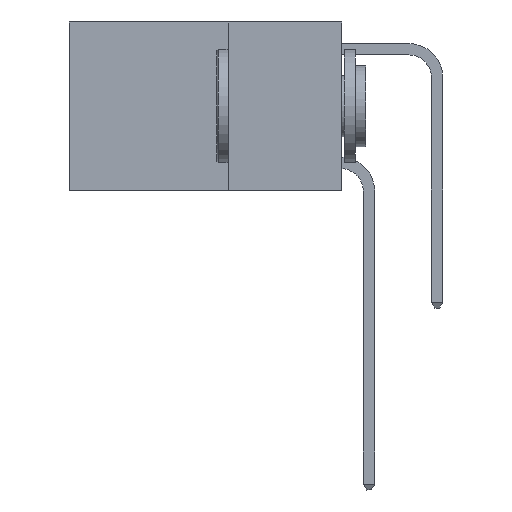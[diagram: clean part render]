
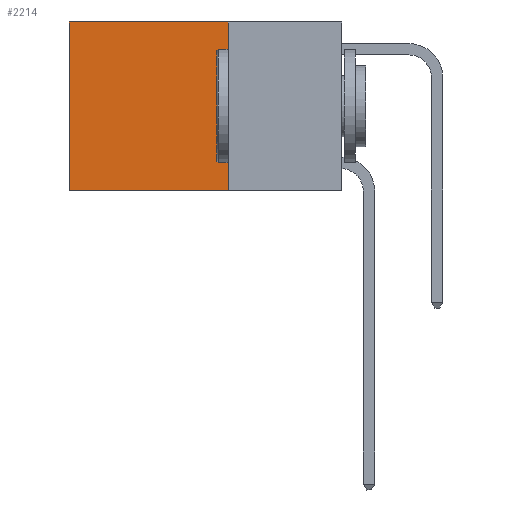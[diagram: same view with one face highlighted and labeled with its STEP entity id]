
A CAD part, left-side view. The second image highlights one B-rep face of the part: STEP entity #2214.
In plain terms, the highlighted planar face has unit normal (-1, 0, 0).
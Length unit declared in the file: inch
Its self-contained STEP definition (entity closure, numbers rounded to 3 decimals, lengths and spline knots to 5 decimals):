
#125 = CARTESIAN_POINT ( 'NONE',  ( 0.2625, 0.25, -0.37 ) ) ;
#917 = CARTESIAN_POINT ( 'NONE',  ( 0.2625, 0.25, 0. ) ) ;
#1165 = LINE ( 'NONE', #2291, #1263 ) ;
#1263 = VECTOR ( 'NONE', #8881, 39.37008 ) ;
#1786 = ORIENTED_EDGE ( 'NONE', *, *, #6537, .F. ) ;
#1971 = LINE ( 'NONE', #917, #6489 ) ;
#2214 = ADVANCED_FACE ( 'NONE', ( #12049 ), #8789, .F. ) ;
#2291 = CARTESIAN_POINT ( 'NONE',  ( 0.2625, 0.25, 0. ) ) ;
#2341 = ORIENTED_EDGE ( 'NONE', *, *, #13356, .T. ) ;
#2422 = CARTESIAN_POINT ( 'NONE',  ( 0.2625, 0.6, 0. ) ) ;
#2552 = VERTEX_POINT ( 'NONE', #7772 ) ;
#3150 = DIRECTION ( 'NONE',  ( 0., 0., -1. ) ) ;
#3165 = AXIS2_PLACEMENT_3D ( 'NONE', #13238, #5432, #12272 ) ;
#4122 = EDGE_CURVE ( 'NONE', #11083, #5513, #1971, .T. ) ;
#4127 = VECTOR ( 'NONE', #8019, 39.37008 ) ;
#4864 = CARTESIAN_POINT ( 'NONE',  ( 0.2625, 0.25, -0.37 ) ) ;
#4879 = LINE ( 'NONE', #2422, #11373 ) ;
#5432 = DIRECTION ( 'NONE',  ( 1., 0., 0. ) ) ;
#5513 = VERTEX_POINT ( 'NONE', #125 ) ;
#6039 = CARTESIAN_POINT ( 'NONE',  ( 0.2625, 0.25, 0. ) ) ;
#6049 = ORIENTED_EDGE ( 'NONE', *, *, #4122, .F. ) ;
#6489 = VECTOR ( 'NONE', #3150, 39.37008 ) ;
#6537 = EDGE_CURVE ( 'NONE', #5513, #2552, #9519, .T. ) ;
#7772 = CARTESIAN_POINT ( 'NONE',  ( 0.2625, 0.6, -0.37 ) ) ;
#7833 = CARTESIAN_POINT ( 'NONE',  ( 0.2625, 0.6, 0. ) ) ;
#8019 = DIRECTION ( 'NONE',  ( 0., 1., 0. ) ) ;
#8645 = EDGE_LOOP ( 'NONE', ( #12099, #1786, #6049, #2341 ) ) ;
#8789 = PLANE ( 'NONE',  #3165 ) ;
#8881 = DIRECTION ( 'NONE',  ( 0., 1., 0. ) ) ;
#9519 = LINE ( 'NONE', #4864, #4127 ) ;
#11047 = VERTEX_POINT ( 'NONE', #7833 ) ;
#11083 = VERTEX_POINT ( 'NONE', #6039 ) ;
#11373 = VECTOR ( 'NONE', #13972, 39.37008 ) ;
#12049 = FACE_OUTER_BOUND ( 'NONE', #8645, .T. ) ;
#12099 = ORIENTED_EDGE ( 'NONE', *, *, #13784, .T. ) ;
#12272 = DIRECTION ( 'NONE',  ( 0., 0., -1. ) ) ;
#13238 = CARTESIAN_POINT ( 'NONE',  ( 0.2625, 0.25, 0. ) ) ;
#13356 = EDGE_CURVE ( 'NONE', #11083, #11047, #1165, .T. ) ;
#13784 = EDGE_CURVE ( 'NONE', #11047, #2552, #4879, .T. ) ;
#13972 = DIRECTION ( 'NONE',  ( 0., 0., -1. ) ) ;
